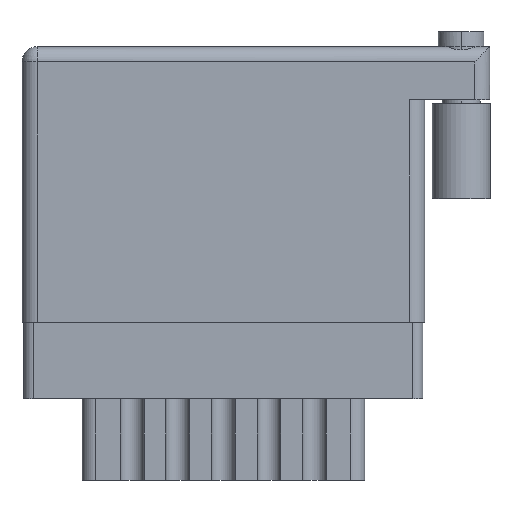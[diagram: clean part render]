
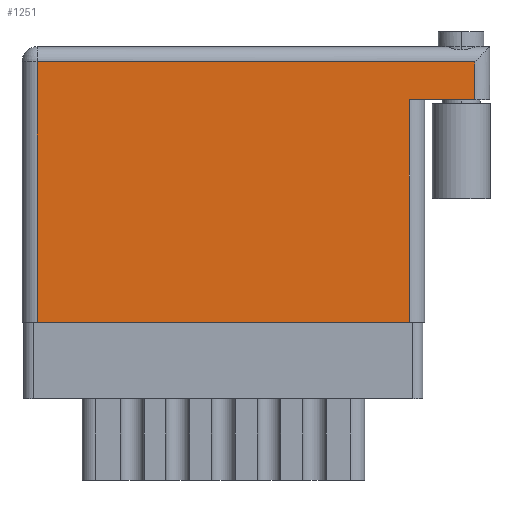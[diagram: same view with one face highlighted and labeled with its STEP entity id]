
A CAD part, front view. The second image highlights one B-rep face of the part: STEP entity #1251.
In plain terms, the highlighted face is planar.
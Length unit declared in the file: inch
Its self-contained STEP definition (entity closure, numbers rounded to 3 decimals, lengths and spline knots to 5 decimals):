
#253 = LINE ( 'NONE', #13440, #11499 ) ;
#369 = VERTEX_POINT ( 'NONE', #683 ) ;
#683 = CARTESIAN_POINT ( 'NONE',  ( 1.489, 0.731, 0. ) ) ;
#827 = VERTEX_POINT ( 'NONE', #11372 ) ;
#1251 = ADVANCED_FACE ( 'NONE', ( #6710 ), #3240, .F. ) ;
#1315 = VERTEX_POINT ( 'NONE', #13604 ) ;
#2862 = VERTEX_POINT ( 'NONE', #13208 ) ;
#3027 = CARTESIAN_POINT ( 'NONE',  ( 0., 0.906, 0. ) ) ;
#3127 = DIRECTION ( 'NONE',  ( -1., 0., 0. ) ) ;
#3240 = PLANE ( 'NONE',  #18354 ) ;
#3261 = VECTOR ( 'NONE', #19037, 39.37008 ) ;
#3375 = EDGE_CURVE ( 'NONE', #2862, #17570, #9203, .T. ) ;
#3761 = EDGE_CURVE ( 'NONE', #369, #827, #253, .T. ) ;
#4956 = CARTESIAN_POINT ( 'NONE',  ( 1.275, 0.731, 0. ) ) ;
#5562 = CARTESIAN_POINT ( 'NONE',  ( 1.275, 0.731, 0. ) ) ;
#5733 = ORIENTED_EDGE ( 'NONE', *, *, #5737, .T. ) ;
#5737 = EDGE_CURVE ( 'NONE', #17570, #7982, #18034, .T. ) ;
#6093 = DIRECTION ( 'NONE',  ( -1., 0., 0. ) ) ;
#6350 = VECTOR ( 'NONE', #8423, 39.37008 ) ;
#6710 = FACE_OUTER_BOUND ( 'NONE', #11960, .T. ) ;
#7305 = ORIENTED_EDGE ( 'NONE', *, *, #3761, .T. ) ;
#7359 = DIRECTION ( 'NONE',  ( 1., 0., 0. ) ) ;
#7490 = LINE ( 'NONE', #20243, #3261 ) ;
#7982 = VERTEX_POINT ( 'NONE', #5562 ) ;
#8277 = DIRECTION ( 'NONE',  ( -1., 0., 0. ) ) ;
#8423 = DIRECTION ( 'NONE',  ( 0., 1., 0. ) ) ;
#8775 = ORIENTED_EDGE ( 'NONE', *, *, #18758, .T. ) ;
#9203 = LINE ( 'NONE', #13727, #21156 ) ;
#11296 = EDGE_CURVE ( 'NONE', #1315, #2862, #7490, .T. ) ;
#11372 = CARTESIAN_POINT ( 'NONE',  ( 1.489, 0.856, 0. ) ) ;
#11499 = VECTOR ( 'NONE', #20053, 39.37008 ) ;
#11958 = ORIENTED_EDGE ( 'NONE', *, *, #3375, .T. ) ;
#11960 = EDGE_LOOP ( 'NONE', ( #11958, #5733, #18389, #7305, #8775, #12055 ) ) ;
#12006 = CARTESIAN_POINT ( 'NONE',  ( 1.275, 0., 0. ) ) ;
#12055 = ORIENTED_EDGE ( 'NONE', *, *, #11296, .T. ) ;
#13208 = CARTESIAN_POINT ( 'NONE',  ( 0.05, 0., 0. ) ) ;
#13284 = DIRECTION ( 'NONE',  ( 0., 0., -1. ) ) ;
#13440 = CARTESIAN_POINT ( 'NONE',  ( 1.489, 0.906, 0. ) ) ;
#13604 = CARTESIAN_POINT ( 'NONE',  ( 0.05, 0.856, 0. ) ) ;
#13727 = CARTESIAN_POINT ( 'NONE',  ( 0., 0., 0. ) ) ;
#13967 = EDGE_CURVE ( 'NONE', #369, #7982, #18107, .T. ) ;
#15443 = VECTOR ( 'NONE', #8277, 39.37008 ) ;
#15705 = VECTOR ( 'NONE', #6093, 39.37008 ) ;
#16033 = CARTESIAN_POINT ( 'NONE',  ( 0., 0.856, 0. ) ) ;
#17570 = VERTEX_POINT ( 'NONE', #12006 ) ;
#18034 = LINE ( 'NONE', #4956, #6350 ) ;
#18107 = LINE ( 'NONE', #18433, #15443 ) ;
#18354 = AXIS2_PLACEMENT_3D ( 'NONE', #3027, #13284, #3127 ) ;
#18389 = ORIENTED_EDGE ( 'NONE', *, *, #13967, .F. ) ;
#18433 = CARTESIAN_POINT ( 'NONE',  ( 1.539, 0.731, 0. ) ) ;
#18758 = EDGE_CURVE ( 'NONE', #827, #1315, #19271, .T. ) ;
#19037 = DIRECTION ( 'NONE',  ( 0., -1., 0. ) ) ;
#19271 = LINE ( 'NONE', #16033, #15705 ) ;
#20053 = DIRECTION ( 'NONE',  ( 0., 1., 0. ) ) ;
#20243 = CARTESIAN_POINT ( 'NONE',  ( 0.05, 0., 0. ) ) ;
#21156 = VECTOR ( 'NONE', #7359, 39.37008 ) ;
